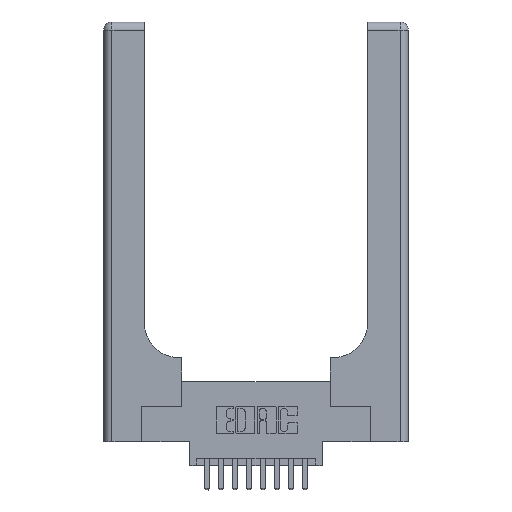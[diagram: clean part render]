
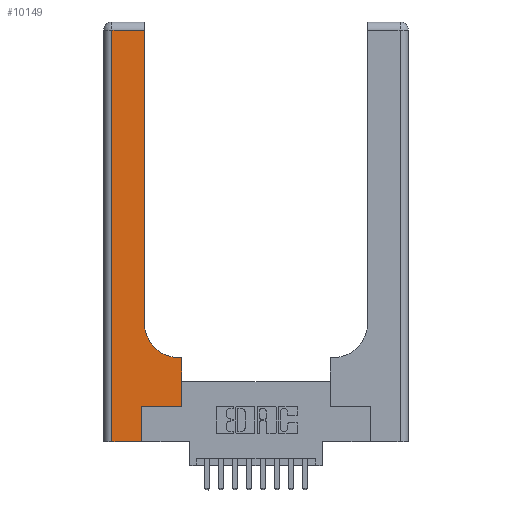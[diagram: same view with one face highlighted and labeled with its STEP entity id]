
A CAD part, top view. The second image highlights one B-rep face of the part: STEP entity #10149.
In plain terms, the highlighted planar face has unit normal (0, 0, 1).
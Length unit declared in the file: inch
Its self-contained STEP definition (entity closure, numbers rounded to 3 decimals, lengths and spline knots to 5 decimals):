
#276 = VERTEX_POINT ( 'NONE', #2405 ) ;
#367 = FACE_OUTER_BOUND ( 'NONE', #14746, .T. ) ;
#486 = ORIENTED_EDGE ( 'NONE', *, *, #5680, .T. ) ;
#767 = CARTESIAN_POINT ( 'NONE',  ( 0.2915, 2.94, 0.37 ) ) ;
#835 = CARTESIAN_POINT ( 'NONE',  ( 0.5585, 0.25, 0.37 ) ) ;
#849 = CARTESIAN_POINT ( 'NONE',  ( 0.5585, 0.25, 0.37 ) ) ;
#1356 = VERTEX_POINT ( 'NONE', #2490 ) ;
#2185 = VECTOR ( 'NONE', #10926, 39.37008 ) ;
#2405 = CARTESIAN_POINT ( 'NONE',  ( 0.06, 0., 0.37 ) ) ;
#2424 = LINE ( 'NONE', #3196, #8789 ) ;
#2490 = CARTESIAN_POINT ( 'NONE',  ( 0.269, 0.25, 0.37 ) ) ;
#2733 = ORIENTED_EDGE ( 'NONE', *, *, #12978, .T. ) ;
#2740 = PLANE ( 'NONE',  #13098 ) ;
#2958 = LINE ( 'NONE', #849, #2185 ) ;
#3178 = EDGE_CURVE ( 'NONE', #13602, #8048, #7931, .T. ) ;
#3196 = CARTESIAN_POINT ( 'NONE',  ( 0., 2.94, 0.37 ) ) ;
#3359 = CARTESIAN_POINT ( 'NONE',  ( 0., 0., 0.37 ) ) ;
#3890 = DIRECTION ( 'NONE',  ( 0., 1., 0. ) ) ;
#3904 = LINE ( 'NONE', #9313, #6491 ) ;
#3937 = VECTOR ( 'NONE', #12365, 39.37008 ) ;
#4015 = EDGE_CURVE ( 'NONE', #8844, #1356, #3904, .T. ) ;
#4179 = VERTEX_POINT ( 'NONE', #835 ) ;
#4514 = VECTOR ( 'NONE', #3890, 39.37008 ) ;
#4592 = VERTEX_POINT ( 'NONE', #14798 ) ;
#4750 = VERTEX_POINT ( 'NONE', #12660 ) ;
#5392 = LINE ( 'NONE', #11844, #11750 ) ;
#5680 = EDGE_CURVE ( 'NONE', #4592, #11313, #7609, .T. ) ;
#5693 = ORIENTED_EDGE ( 'NONE', *, *, #3178, .T. ) ;
#5734 = DIRECTION ( 'NONE',  ( 0., 0., -1. ) ) ;
#6355 = AXIS2_PLACEMENT_3D ( 'NONE', #13310, #5734, #14576 ) ;
#6491 = VECTOR ( 'NONE', #11841, 39.37008 ) ;
#6560 = CARTESIAN_POINT ( 'NONE',  ( 0., 3., 0.37 ) ) ;
#6822 = DIRECTION ( 'NONE',  ( 1., 0., 0. ) ) ;
#7352 = LINE ( 'NONE', #16085, #3937 ) ;
#7609 = LINE ( 'NONE', #14438, #13508 ) ;
#7747 = CARTESIAN_POINT ( 'NONE',  ( 0.269, 0., 0.37 ) ) ;
#7867 = DIRECTION ( 'NONE',  ( -1., 0., 0. ) ) ;
#7931 = LINE ( 'NONE', #8963, #4514 ) ;
#8048 = VERTEX_POINT ( 'NONE', #767 ) ;
#8425 = CARTESIAN_POINT ( 'NONE',  ( 0.2915, 0.85, 0.37 ) ) ;
#8599 = CIRCLE ( 'NONE', #6355, 0.25 ) ;
#8789 = VECTOR ( 'NONE', #9536, 39.37008 ) ;
#8844 = VERTEX_POINT ( 'NONE', #7747 ) ;
#8873 = ORIENTED_EDGE ( 'NONE', *, *, #12038, .T. ) ;
#8893 = ORIENTED_EDGE ( 'NONE', *, *, #14344, .T. ) ;
#8963 = CARTESIAN_POINT ( 'NONE',  ( 0.2915, 3., 0.37 ) ) ;
#9069 = CARTESIAN_POINT ( 'NONE',  ( 0.5415, 0.6, 0.37 ) ) ;
#9313 = CARTESIAN_POINT ( 'NONE',  ( 0.269, 0., 0.37 ) ) ;
#9376 = LINE ( 'NONE', #3359, #15662 ) ;
#9536 = DIRECTION ( 'NONE',  ( -1., 0., 0. ) ) ;
#9666 = ORIENTED_EDGE ( 'NONE', *, *, #4015, .T. ) ;
#10149 = ADVANCED_FACE ( 'NONE', ( #367 ), #2740, .F. ) ;
#10926 = DIRECTION ( 'NONE',  ( 0., 1., 0. ) ) ;
#10966 = DIRECTION ( 'NONE',  ( 1., 0., 0. ) ) ;
#11313 = VERTEX_POINT ( 'NONE', #9069 ) ;
#11750 = VECTOR ( 'NONE', #6822, 39.37008 ) ;
#11841 = DIRECTION ( 'NONE',  ( 0., 1., 0. ) ) ;
#11844 = CARTESIAN_POINT ( 'NONE',  ( 0.269, 0.25, 0.37 ) ) ;
#11967 = DIRECTION ( 'NONE',  ( -1., 0., 0. ) ) ;
#12038 = EDGE_CURVE ( 'NONE', #1356, #4179, #5392, .T. ) ;
#12224 = EDGE_CURVE ( 'NONE', #276, #8844, #9376, .T. ) ;
#12365 = DIRECTION ( 'NONE',  ( 0., -1., 0. ) ) ;
#12660 = CARTESIAN_POINT ( 'NONE',  ( 0.06, 2.94, 0.37 ) ) ;
#12745 = EDGE_CURVE ( 'NONE', #11313, #13602, #8599, .T. ) ;
#12978 = EDGE_CURVE ( 'NONE', #8048, #4750, #2424, .T. ) ;
#13098 = AXIS2_PLACEMENT_3D ( 'NONE', #6560, #15386, #7867 ) ;
#13310 = CARTESIAN_POINT ( 'NONE',  ( 0.5415, 0.85, 0.37 ) ) ;
#13342 = ORIENTED_EDGE ( 'NONE', *, *, #14247, .T. ) ;
#13508 = VECTOR ( 'NONE', #11967, 39.37008 ) ;
#13602 = VERTEX_POINT ( 'NONE', #8425 ) ;
#13807 = ORIENTED_EDGE ( 'NONE', *, *, #12224, .T. ) ;
#14247 = EDGE_CURVE ( 'NONE', #4179, #4592, #2958, .T. ) ;
#14344 = EDGE_CURVE ( 'NONE', #4750, #276, #7352, .T. ) ;
#14438 = CARTESIAN_POINT ( 'NONE',  ( 0.2915, 0.6, 0.37 ) ) ;
#14576 = DIRECTION ( 'NONE',  ( 1., 0., 0. ) ) ;
#14746 = EDGE_LOOP ( 'NONE', ( #5693, #2733, #8893, #13807, #9666, #8873, #13342, #486, #15550 ) ) ;
#14798 = CARTESIAN_POINT ( 'NONE',  ( 0.5585, 0.6, 0.37 ) ) ;
#15386 = DIRECTION ( 'NONE',  ( 0., 0., -1. ) ) ;
#15550 = ORIENTED_EDGE ( 'NONE', *, *, #12745, .T. ) ;
#15662 = VECTOR ( 'NONE', #10966, 39.37008 ) ;
#16085 = CARTESIAN_POINT ( 'NONE',  ( 0.06, 3., 0.37 ) ) ;
